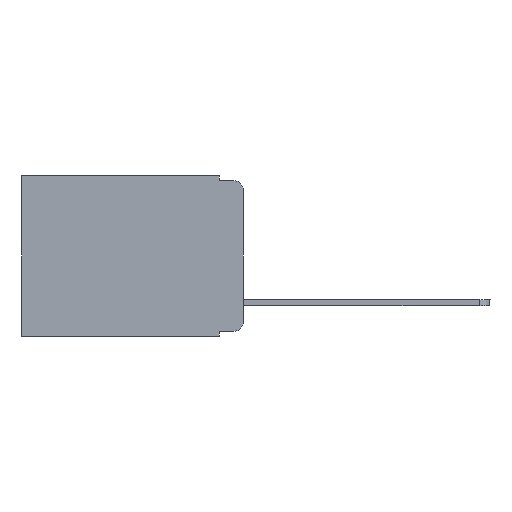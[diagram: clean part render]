
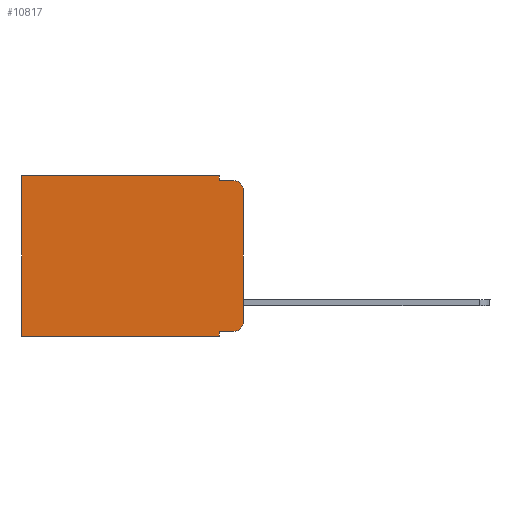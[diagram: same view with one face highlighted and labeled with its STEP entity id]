
A CAD part, left-side view. The second image highlights one B-rep face of the part: STEP entity #10817.
In plain terms, the highlighted planar face has unit normal (-1, 0, 0).
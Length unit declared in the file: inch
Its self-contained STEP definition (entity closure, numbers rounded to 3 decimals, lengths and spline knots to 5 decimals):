
#30 = VECTOR ( 'NONE', #2620, 39.37008 ) ;
#54 = EDGE_CURVE ( 'NONE', #1372, #10630, #4577, .T. ) ;
#87 = DIRECTION ( 'NONE',  ( 0., 0., -1. ) ) ;
#170 = ORIENTED_EDGE ( 'NONE', *, *, #7604, .T. ) ;
#189 = EDGE_CURVE ( 'NONE', #8629, #10630, #3245, .T. ) ;
#263 = LINE ( 'NONE', #7303, #7876 ) ;
#331 = CARTESIAN_POINT ( 'NONE',  ( 0.298, 0.051, -0.01 ) ) ;
#433 = CARTESIAN_POINT ( 'NONE',  ( 0.298, 0.02, -0.333 ) ) ;
#689 = VECTOR ( 'NONE', #7007, 39.37008 ) ;
#702 = AXIS2_PLACEMENT_3D ( 'NONE', #5564, #2907, #87 ) ;
#773 = ORIENTED_EDGE ( 'NONE', *, *, #54, .T. ) ;
#793 = LINE ( 'NONE', #4362, #689 ) ;
#936 = CARTESIAN_POINT ( 'NONE',  ( 0.298, 0.051, 0. ) ) ;
#1269 = EDGE_CURVE ( 'NONE', #3153, #6234, #10707, .T. ) ;
#1369 = VECTOR ( 'NONE', #1841, 39.37008 ) ;
#1370 = CARTESIAN_POINT ( 'NONE',  ( 0.298, 0.02, -0.03 ) ) ;
#1372 = VERTEX_POINT ( 'NONE', #433 ) ;
#1431 = CARTESIAN_POINT ( 'NONE',  ( 0.298, 0., -0.03 ) ) ;
#1460 = VECTOR ( 'NONE', #8287, 39.37008 ) ;
#1810 = EDGE_CURVE ( 'NONE', #2074, #6976, #7846, .T. ) ;
#1841 = DIRECTION ( 'NONE',  ( 0., 0., -1. ) ) ;
#1983 = FACE_OUTER_BOUND ( 'NONE', #9127, .T. ) ;
#2074 = VERTEX_POINT ( 'NONE', #10257 ) ;
#2094 = DIRECTION ( 'NONE',  ( 0., 0., -1. ) ) ;
#2125 = DIRECTION ( 'NONE',  ( 0., 1., 0. ) ) ;
#2272 = ORIENTED_EDGE ( 'NONE', *, *, #9203, .F. ) ;
#2558 = CARTESIAN_POINT ( 'NONE',  ( 0.298, 0., -0.313 ) ) ;
#2574 = CARTESIAN_POINT ( 'NONE',  ( 0.298, 0.473, 0. ) ) ;
#2620 = DIRECTION ( 'NONE',  ( 0., 0., -1. ) ) ;
#2772 = ORIENTED_EDGE ( 'NONE', *, *, #189, .F. ) ;
#2907 = DIRECTION ( 'NONE',  ( 1., 0., 0. ) ) ;
#3149 = CARTESIAN_POINT ( 'NONE',  ( 0.298, 0.473, -0.343 ) ) ;
#3153 = VERTEX_POINT ( 'NONE', #936 ) ;
#3245 = LINE ( 'NONE', #7749, #10151 ) ;
#3404 = ORIENTED_EDGE ( 'NONE', *, *, #1810, .F. ) ;
#3660 = VERTEX_POINT ( 'NONE', #3991 ) ;
#3692 = EDGE_CURVE ( 'NONE', #2074, #1372, #7508, .T. ) ;
#3701 = CARTESIAN_POINT ( 'NONE',  ( 0.298, 0.051, -0.343 ) ) ;
#3991 = CARTESIAN_POINT ( 'NONE',  ( 0.298, 0.02, -0.01 ) ) ;
#4362 = CARTESIAN_POINT ( 'NONE',  ( 0.298, 0.473, 0. ) ) ;
#4473 = VECTOR ( 'NONE', #7340, 39.37008 ) ;
#4566 = ORIENTED_EDGE ( 'NONE', *, *, #1269, .F. ) ;
#4577 = CIRCLE ( 'NONE', #11041, 0.02 ) ;
#4738 = CARTESIAN_POINT ( 'NONE',  ( 0.298, 0.051, -0.333 ) ) ;
#4797 = DIRECTION ( 'NONE',  ( -1., 0., 0. ) ) ;
#4840 = EDGE_CURVE ( 'NONE', #6976, #5858, #263, .T. ) ;
#4945 = ORIENTED_EDGE ( 'NONE', *, *, #8156, .T. ) ;
#5005 = CARTESIAN_POINT ( 'NONE',  ( 0.298, 0., 0. ) ) ;
#5234 = CARTESIAN_POINT ( 'NONE',  ( 0.298, 0.051, 0. ) ) ;
#5522 = LINE ( 'NONE', #7324, #1460 ) ;
#5523 = VERTEX_POINT ( 'NONE', #2574 ) ;
#5560 = DIRECTION ( 'NONE',  ( -1., 0., 0. ) ) ;
#5564 = CARTESIAN_POINT ( 'NONE',  ( 0.298, 0., 0. ) ) ;
#5858 = VERTEX_POINT ( 'NONE', #3149 ) ;
#6234 = VERTEX_POINT ( 'NONE', #331 ) ;
#6517 = LINE ( 'NONE', #5005, #11481 ) ;
#6947 = ORIENTED_EDGE ( 'NONE', *, *, #4840, .F. ) ;
#6976 = VERTEX_POINT ( 'NONE', #3701 ) ;
#7007 = DIRECTION ( 'NONE',  ( 0., 0., -1. ) ) ;
#7050 = EDGE_CURVE ( 'NONE', #8629, #3660, #9264, .T. ) ;
#7303 = CARTESIAN_POINT ( 'NONE',  ( 0.298, 0., -0.343 ) ) ;
#7324 = CARTESIAN_POINT ( 'NONE',  ( 0.298, 0.051, -0.01 ) ) ;
#7340 = DIRECTION ( 'NONE',  ( 0., -1., 0. ) ) ;
#7354 = DIRECTION ( 'NONE',  ( 0., 1., 0. ) ) ;
#7508 = LINE ( 'NONE', #4738, #4473 ) ;
#7604 = EDGE_CURVE ( 'NONE', #3153, #5523, #6517, .T. ) ;
#7680 = ORIENTED_EDGE ( 'NONE', *, *, #7050, .T. ) ;
#7749 = CARTESIAN_POINT ( 'NONE',  ( 0.298, 0., 0. ) ) ;
#7846 = LINE ( 'NONE', #9750, #1369 ) ;
#7876 = VECTOR ( 'NONE', #7354, 39.37008 ) ;
#8156 = EDGE_CURVE ( 'NONE', #5523, #5858, #793, .T. ) ;
#8287 = DIRECTION ( 'NONE',  ( 0., -1., 0. ) ) ;
#8629 = VERTEX_POINT ( 'NONE', #1431 ) ;
#8964 = CARTESIAN_POINT ( 'NONE',  ( 0.298, 0.02, -0.313 ) ) ;
#9127 = EDGE_LOOP ( 'NONE', ( #2772, #7680, #2272, #4566, #170, #4945, #6947, #3404, #9749, #773 ) ) ;
#9203 = EDGE_CURVE ( 'NONE', #6234, #3660, #5522, .T. ) ;
#9258 = DIRECTION ( 'NONE',  ( 0., 0., -1. ) ) ;
#9264 = CIRCLE ( 'NONE', #10015, 0.02 ) ;
#9749 = ORIENTED_EDGE ( 'NONE', *, *, #3692, .T. ) ;
#9750 = CARTESIAN_POINT ( 'NONE',  ( 0.298, 0.051, 0. ) ) ;
#10006 = DIRECTION ( 'NONE',  ( 0., 0., -1. ) ) ;
#10015 = AXIS2_PLACEMENT_3D ( 'NONE', #1370, #4797, #10006 ) ;
#10151 = VECTOR ( 'NONE', #9258, 39.37008 ) ;
#10257 = CARTESIAN_POINT ( 'NONE',  ( 0.298, 0.051, -0.333 ) ) ;
#10599 = PLANE ( 'NONE',  #702 ) ;
#10630 = VERTEX_POINT ( 'NONE', #2558 ) ;
#10707 = LINE ( 'NONE', #5234, #30 ) ;
#10817 = ADVANCED_FACE ( 'NONE', ( #1983 ), #10599, .F. ) ;
#11041 = AXIS2_PLACEMENT_3D ( 'NONE', #8964, #5560, #2094 ) ;
#11481 = VECTOR ( 'NONE', #2125, 39.37008 ) ;
